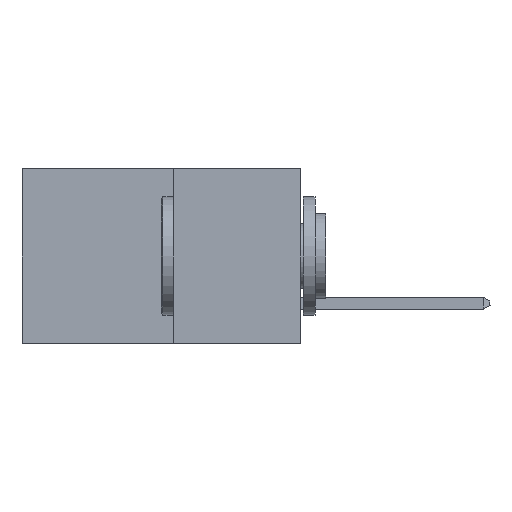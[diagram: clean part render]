
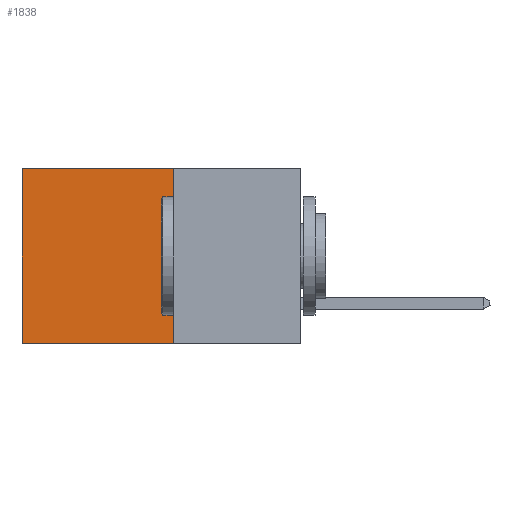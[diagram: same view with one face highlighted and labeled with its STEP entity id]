
A CAD part, left-side view. The second image highlights one B-rep face of the part: STEP entity #1838.
In plain terms, the highlighted planar face has unit normal (-1, 0, 0).
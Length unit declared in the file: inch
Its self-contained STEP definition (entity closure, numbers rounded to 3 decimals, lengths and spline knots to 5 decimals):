
#559 = CARTESIAN_POINT ( 'NONE',  ( 0.277, 0.27, -0.37 ) ) ;
#1393 = CARTESIAN_POINT ( 'NONE',  ( 0.277, 0.59, 0. ) ) ;
#1601 = VERTEX_POINT ( 'NONE', #1393 ) ;
#1838 = ADVANCED_FACE ( 'NONE', ( #25479 ), #27893, .F. ) ;
#4611 = CARTESIAN_POINT ( 'NONE',  ( 0.277, 0.59, -0.37 ) ) ;
#4883 = VERTEX_POINT ( 'NONE', #28065 ) ;
#5495 = VECTOR ( 'NONE', #24679, 39.37008 ) ;
#6235 = EDGE_CURVE ( 'NONE', #4883, #20109, #18751, .T. ) ;
#6771 = VERTEX_POINT ( 'NONE', #4611 ) ;
#8366 = ORIENTED_EDGE ( 'NONE', *, *, #26508, .F. ) ;
#10457 = EDGE_LOOP ( 'NONE', ( #14619, #8366, #26353, #16930 ) ) ;
#10844 = CARTESIAN_POINT ( 'NONE',  ( 0.277, 0.27, 0. ) ) ;
#12425 = LINE ( 'NONE', #10844, #5495 ) ;
#12776 = CARTESIAN_POINT ( 'NONE',  ( 0.277, 0.59, -0.37 ) ) ;
#14594 = EDGE_CURVE ( 'NONE', #1601, #6771, #24880, .T. ) ;
#14619 = ORIENTED_EDGE ( 'NONE', *, *, #14594, .T. ) ;
#15099 = DIRECTION ( 'NONE',  ( 0., 0., -1. ) ) ;
#15191 = DIRECTION ( 'NONE',  ( 0., 0., -1. ) ) ;
#15448 = DIRECTION ( 'NONE',  ( 1., 0., 0. ) ) ;
#15896 = VECTOR ( 'NONE', #17666, 39.37008 ) ;
#16748 = EDGE_CURVE ( 'NONE', #4883, #1601, #12425, .T. ) ;
#16879 = DIRECTION ( 'NONE',  ( 0., 0., -1. ) ) ;
#16930 = ORIENTED_EDGE ( 'NONE', *, *, #16748, .T. ) ;
#17666 = DIRECTION ( 'NONE',  ( 0., 1., 0. ) ) ;
#18746 = VECTOR ( 'NONE', #15099, 39.37008 ) ;
#18751 = LINE ( 'NONE', #559, #24884 ) ;
#20109 = VERTEX_POINT ( 'NONE', #24745 ) ;
#20498 = AXIS2_PLACEMENT_3D ( 'NONE', #28190, #15448, #15191 ) ;
#24679 = DIRECTION ( 'NONE',  ( 0., 1., 0. ) ) ;
#24745 = CARTESIAN_POINT ( 'NONE',  ( 0.277, 0.27, -0.37 ) ) ;
#24880 = LINE ( 'NONE', #12776, #18746 ) ;
#24884 = VECTOR ( 'NONE', #16879, 39.37008 ) ;
#25479 = FACE_OUTER_BOUND ( 'NONE', #10457, .T. ) ;
#26353 = ORIENTED_EDGE ( 'NONE', *, *, #6235, .F. ) ;
#26508 = EDGE_CURVE ( 'NONE', #20109, #6771, #28172, .T. ) ;
#26856 = CARTESIAN_POINT ( 'NONE',  ( 0.277, 0.27, -0.37 ) ) ;
#27893 = PLANE ( 'NONE',  #20498 ) ;
#28065 = CARTESIAN_POINT ( 'NONE',  ( 0.277, 0.27, 0. ) ) ;
#28172 = LINE ( 'NONE', #26856, #15896 ) ;
#28190 = CARTESIAN_POINT ( 'NONE',  ( 0.277, 0.27, -0.37 ) ) ;
